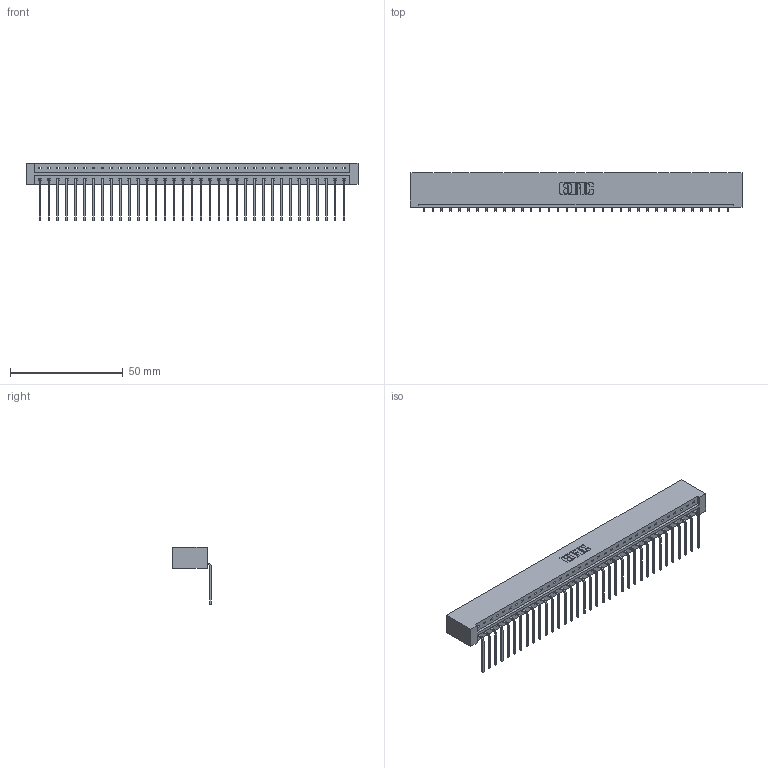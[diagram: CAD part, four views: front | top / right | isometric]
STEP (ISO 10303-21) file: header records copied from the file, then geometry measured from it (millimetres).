
FILE_DESCRIPTION (( 'STEP AP203' ), '1' );
FILE_NAME ('833-035-559-101.STEP', '2020-06-03T01:11:17', ( '' ), ( '' ), 'SwSTEP 2.0', 'SolidWorks 2020', '' );
FILE_SCHEMA (( 'CONFIG_CONTROL_DESIGN' ));
Length unit declared in the file: inch
Products named in the file (3): 833 Part_Lugless; 345-292-001_558 559 Tail - 1; 833-035-559-101
Assembly tree (36 placements, depth 2):
  833-035-559-101
    833 Part_Lugless
    345-292-001_558 559 Tail - 1  x35
Bounding box: 146.94 x 17.09 x 25.53 mm (x, y, z)
Volume: 15455.4 mm3; surface area: 17348.2 mm2
Topology: 36 solids, 36 shells, 2206 faces, 6657 edges, 4390 vertices
Faces by surface type: plane 1606, cylinder 600
Entity records: 22109 total; most frequent: CARTESIAN_POINT 3823, ORIENTED_EDGE 3794, DIRECTION 3231, EDGE_CURVE 1897, VECTOR 1777, LINE 1777, VERTEX_POINT 1262, AXIS2_PLACEMENT_3D 727
